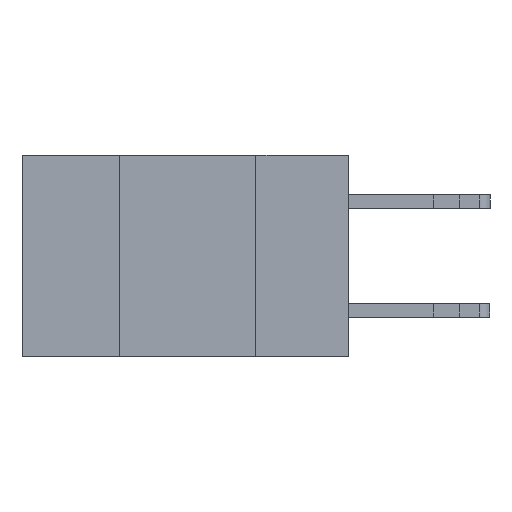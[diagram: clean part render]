
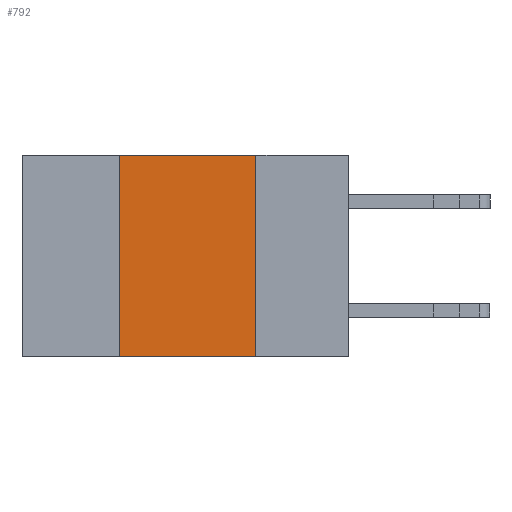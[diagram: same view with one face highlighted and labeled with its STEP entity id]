
A CAD part, left-side view. The second image highlights one B-rep face of the part: STEP entity #792.
In plain terms, the highlighted planar face has unit normal (-1, 0, 0).
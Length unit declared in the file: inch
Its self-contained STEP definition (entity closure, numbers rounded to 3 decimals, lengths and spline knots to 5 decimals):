
#545 = CARTESIAN_POINT ( 'NONE',  ( 0., 0.6, 0. ) ) ;
#792 = ADVANCED_FACE ( 'NONE', ( #17824 ), #14842, .F. ) ;
#1229 = CARTESIAN_POINT ( 'NONE',  ( 0., 0.6, -0.37 ) ) ;
#2180 = LINE ( 'NONE', #14143, #11238 ) ;
#3323 = ORIENTED_EDGE ( 'NONE', *, *, #4601, .F. ) ;
#3850 = DIRECTION ( 'NONE',  ( 0., -1., 0. ) ) ;
#4601 = EDGE_CURVE ( 'NONE', #14320, #15730, #22568, .T. ) ;
#5895 = AXIS2_PLACEMENT_3D ( 'NONE', #545, #21817, #7139 ) ;
#6944 = CARTESIAN_POINT ( 'NONE',  ( 0., 0.17, -0.37 ) ) ;
#7139 = DIRECTION ( 'NONE',  ( 0., 0., -1. ) ) ;
#8805 = CARTESIAN_POINT ( 'NONE',  ( 0., 0.42, -0.37 ) ) ;
#9237 = DIRECTION ( 'NONE',  ( 0., 0., -1. ) ) ;
#10245 = EDGE_LOOP ( 'NONE', ( #3323, #13488, #18295, #11536 ) ) ;
#10283 = DIRECTION ( 'NONE',  ( 0., -1., 0. ) ) ;
#11238 = VECTOR ( 'NONE', #12333, 39.37008 ) ;
#11536 = ORIENTED_EDGE ( 'NONE', *, *, #11849, .T. ) ;
#11849 = EDGE_CURVE ( 'NONE', #15065, #15730, #21893, .T. ) ;
#12333 = DIRECTION ( 'NONE',  ( 0., 0., 1. ) ) ;
#13488 = ORIENTED_EDGE ( 'NONE', *, *, #20368, .F. ) ;
#14143 = CARTESIAN_POINT ( 'NONE',  ( 0., 0.42, 0. ) ) ;
#14320 = VERTEX_POINT ( 'NONE', #15642 ) ;
#14512 = LINE ( 'NONE', #16384, #19902 ) ;
#14842 = PLANE ( 'NONE',  #5895 ) ;
#15065 = VERTEX_POINT ( 'NONE', #8805 ) ;
#15642 = CARTESIAN_POINT ( 'NONE',  ( 0., 0.17, 0. ) ) ;
#15730 = VERTEX_POINT ( 'NONE', #6944 ) ;
#16384 = CARTESIAN_POINT ( 'NONE',  ( 0., 0.6, 0. ) ) ;
#16466 = CARTESIAN_POINT ( 'NONE',  ( 0., 0.42, 0. ) ) ;
#17208 = VERTEX_POINT ( 'NONE', #16466 ) ;
#17443 = CARTESIAN_POINT ( 'NONE',  ( 0., 0.17, 0. ) ) ;
#17713 = VECTOR ( 'NONE', #9237, 39.37008 ) ;
#17824 = FACE_OUTER_BOUND ( 'NONE', #10245, .T. ) ;
#18295 = ORIENTED_EDGE ( 'NONE', *, *, #18796, .F. ) ;
#18796 = EDGE_CURVE ( 'NONE', #15065, #17208, #2180, .T. ) ;
#19902 = VECTOR ( 'NONE', #3850, 39.37008 ) ;
#20368 = EDGE_CURVE ( 'NONE', #17208, #14320, #14512, .T. ) ;
#21817 = DIRECTION ( 'NONE',  ( 1., 0., 0. ) ) ;
#21893 = LINE ( 'NONE', #1229, #22474 ) ;
#22474 = VECTOR ( 'NONE', #10283, 39.37008 ) ;
#22568 = LINE ( 'NONE', #17443, #17713 ) ;
